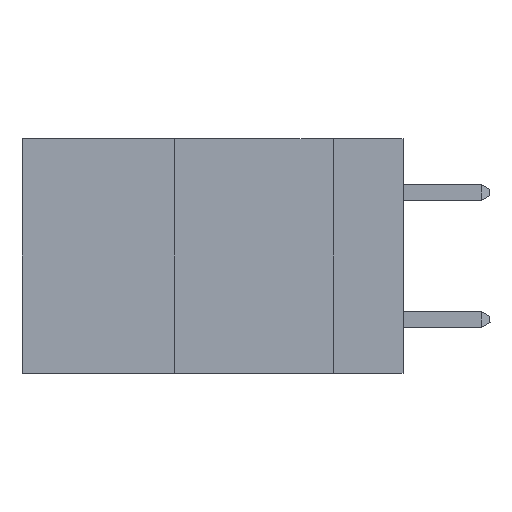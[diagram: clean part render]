
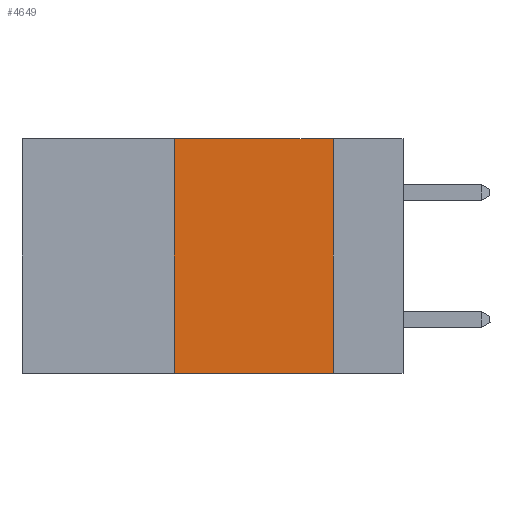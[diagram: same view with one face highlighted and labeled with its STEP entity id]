
A CAD part, left-side view. The second image highlights one B-rep face of the part: STEP entity #4649.
In plain terms, the highlighted planar face has unit normal (-1, 0, 0).
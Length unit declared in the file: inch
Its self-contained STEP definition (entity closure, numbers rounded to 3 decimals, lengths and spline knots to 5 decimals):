
#1167 = VERTEX_POINT ( 'NONE', #16843 ) ;
#1299 = DIRECTION ( 'NONE',  ( 0., -1., 0. ) ) ;
#3257 = VECTOR ( 'NONE', #26794, 39.37008 ) ;
#4516 = VERTEX_POINT ( 'NONE', #30285 ) ;
#4649 = ADVANCED_FACE ( 'NONE', ( #25526 ), #24223, .F. ) ;
#5048 = EDGE_CURVE ( 'NONE', #1167, #16290, #30466, .T. ) ;
#5638 = EDGE_CURVE ( 'NONE', #4516, #18006, #25950, .T. ) ;
#6075 = ORIENTED_EDGE ( 'NONE', *, *, #5048, .F. ) ;
#6133 = VECTOR ( 'NONE', #29402, 39.37008 ) ;
#6192 = DIRECTION ( 'NONE',  ( 1., 0., 0. ) ) ;
#8651 = CARTESIAN_POINT ( 'NONE',  ( 0., 0.11, 0. ) ) ;
#10483 = VECTOR ( 'NONE', #26484, 39.37008 ) ;
#11981 = ORIENTED_EDGE ( 'NONE', *, *, #25295, .F. ) ;
#13521 = CARTESIAN_POINT ( 'NONE',  ( 0., 0.6, 0. ) ) ;
#15791 = CARTESIAN_POINT ( 'NONE',  ( 0., 0.6, 0. ) ) ;
#16236 = ORIENTED_EDGE ( 'NONE', *, *, #5638, .T. ) ;
#16290 = VERTEX_POINT ( 'NONE', #24292 ) ;
#16843 = CARTESIAN_POINT ( 'NONE',  ( 0., 0.36, 0. ) ) ;
#18006 = VERTEX_POINT ( 'NONE', #19366 ) ;
#19366 = CARTESIAN_POINT ( 'NONE',  ( 0., 0.11, -0.37 ) ) ;
#21448 = ORIENTED_EDGE ( 'NONE', *, *, #23861, .F. ) ;
#23185 = AXIS2_PLACEMENT_3D ( 'NONE', #13521, #6192, #45346 ) ;
#23861 = EDGE_CURVE ( 'NONE', #4516, #1167, #34448, .T. ) ;
#24223 = PLANE ( 'NONE',  #23185 ) ;
#24292 = CARTESIAN_POINT ( 'NONE',  ( 0., 0.11, 0. ) ) ;
#24872 = VECTOR ( 'NONE', #1299, 39.37008 ) ;
#25295 = EDGE_CURVE ( 'NONE', #16290, #18006, #29370, .T. ) ;
#25526 = FACE_OUTER_BOUND ( 'NONE', #33500, .T. ) ;
#25950 = LINE ( 'NONE', #29428, #24872 ) ;
#26484 = DIRECTION ( 'NONE',  ( 0., 0., -1. ) ) ;
#26794 = DIRECTION ( 'NONE',  ( 0., -1., 0. ) ) ;
#29370 = LINE ( 'NONE', #8651, #10483 ) ;
#29402 = DIRECTION ( 'NONE',  ( 0., 0., 1. ) ) ;
#29428 = CARTESIAN_POINT ( 'NONE',  ( 0., 0.6, -0.37 ) ) ;
#30285 = CARTESIAN_POINT ( 'NONE',  ( 0., 0.36, -0.37 ) ) ;
#30466 = LINE ( 'NONE', #15791, #3257 ) ;
#33500 = EDGE_LOOP ( 'NONE', ( #11981, #6075, #21448, #16236 ) ) ;
#34448 = LINE ( 'NONE', #35894, #6133 ) ;
#35894 = CARTESIAN_POINT ( 'NONE',  ( 0., 0.36, 0. ) ) ;
#45346 = DIRECTION ( 'NONE',  ( 0., 0., -1. ) ) ;
